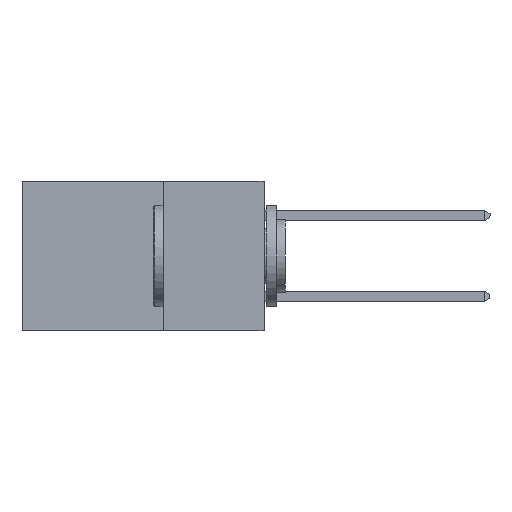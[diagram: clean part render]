
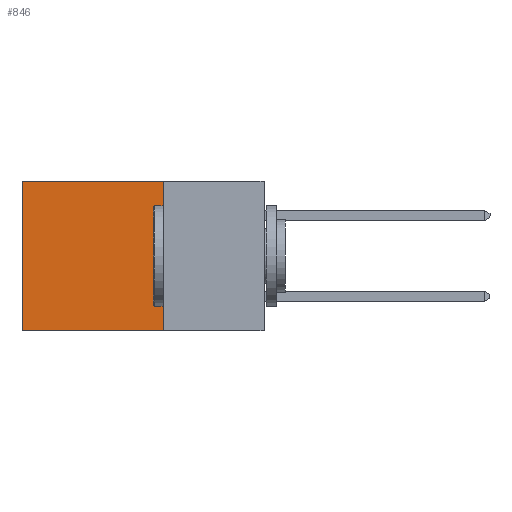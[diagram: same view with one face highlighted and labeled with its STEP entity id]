
A CAD part, left-side view. The second image highlights one B-rep face of the part: STEP entity #846.
In plain terms, the highlighted planar face has unit normal (-1, 0, 0).
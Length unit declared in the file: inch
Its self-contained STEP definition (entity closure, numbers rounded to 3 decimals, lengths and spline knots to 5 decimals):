
#111 = EDGE_LOOP ( 'NONE', ( #4742, #7046, #154, #2693 ) ) ;
#154 = ORIENTED_EDGE ( 'NONE', *, *, #5476, .F. ) ;
#168 = VECTOR ( 'NONE', #11270, 39.37008 ) ;
#356 = VERTEX_POINT ( 'NONE', #901 ) ;
#451 = CARTESIAN_POINT ( 'NONE',  ( 0.298, 0.25, 0. ) ) ;
#581 = VERTEX_POINT ( 'NONE', #1706 ) ;
#846 = ADVANCED_FACE ( 'NONE', ( #2479 ), #5460, .F. ) ;
#901 = CARTESIAN_POINT ( 'NONE',  ( 0.298, 0.6, 0. ) ) ;
#1303 = CARTESIAN_POINT ( 'NONE',  ( 0.298, 0.6, 0. ) ) ;
#1706 = CARTESIAN_POINT ( 'NONE',  ( 0.298, 0.25, -0.37 ) ) ;
#2085 = CARTESIAN_POINT ( 'NONE',  ( 0.298, 0.25, 0. ) ) ;
#2201 = DIRECTION ( 'NONE',  ( 0., 1., 0. ) ) ;
#2224 = DIRECTION ( 'NONE',  ( 0., 0., -1. ) ) ;
#2479 = FACE_OUTER_BOUND ( 'NONE', #111, .T. ) ;
#2693 = ORIENTED_EDGE ( 'NONE', *, *, #5969, .T. ) ;
#2756 = AXIS2_PLACEMENT_3D ( 'NONE', #6569, #8774, #3655 ) ;
#2988 = LINE ( 'NONE', #9340, #168 ) ;
#3241 = EDGE_CURVE ( 'NONE', #581, #6634, #3442, .T. ) ;
#3442 = LINE ( 'NONE', #10986, #7775 ) ;
#3655 = DIRECTION ( 'NONE',  ( 0., 0., -1. ) ) ;
#3914 = VECTOR ( 'NONE', #2201, 39.37008 ) ;
#4172 = DIRECTION ( 'NONE',  ( 0., 1., 0. ) ) ;
#4339 = EDGE_CURVE ( 'NONE', #356, #6634, #5686, .T. ) ;
#4742 = ORIENTED_EDGE ( 'NONE', *, *, #4339, .T. ) ;
#5261 = VERTEX_POINT ( 'NONE', #2085 ) ;
#5441 = VECTOR ( 'NONE', #2224, 39.37008 ) ;
#5460 = PLANE ( 'NONE',  #2756 ) ;
#5476 = EDGE_CURVE ( 'NONE', #5261, #581, #2988, .T. ) ;
#5686 = LINE ( 'NONE', #1303, #5441 ) ;
#5969 = EDGE_CURVE ( 'NONE', #5261, #356, #10688, .T. ) ;
#6569 = CARTESIAN_POINT ( 'NONE',  ( 0.298, 0.25, 0. ) ) ;
#6634 = VERTEX_POINT ( 'NONE', #7139 ) ;
#7046 = ORIENTED_EDGE ( 'NONE', *, *, #3241, .F. ) ;
#7139 = CARTESIAN_POINT ( 'NONE',  ( 0.298, 0.6, -0.37 ) ) ;
#7775 = VECTOR ( 'NONE', #4172, 39.37008 ) ;
#8774 = DIRECTION ( 'NONE',  ( 1., 0., 0. ) ) ;
#9340 = CARTESIAN_POINT ( 'NONE',  ( 0.298, 0.25, 0. ) ) ;
#10688 = LINE ( 'NONE', #451, #3914 ) ;
#10986 = CARTESIAN_POINT ( 'NONE',  ( 0.298, 0.25, -0.37 ) ) ;
#11270 = DIRECTION ( 'NONE',  ( 0., 0., -1. ) ) ;
